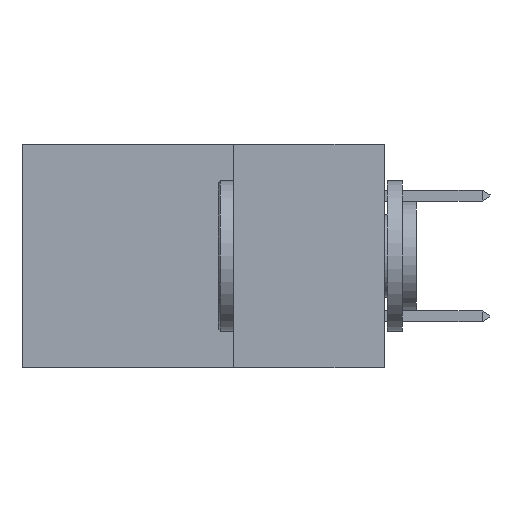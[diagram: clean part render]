
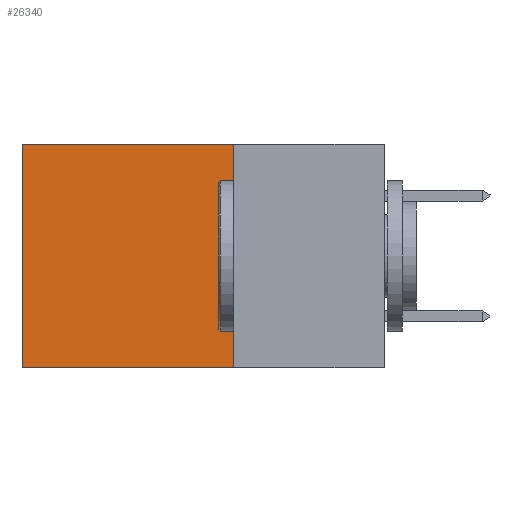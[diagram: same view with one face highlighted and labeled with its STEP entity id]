
A CAD part, left-side view. The second image highlights one B-rep face of the part: STEP entity #26340.
In plain terms, the highlighted planar face has unit normal (-1, 0, 0).
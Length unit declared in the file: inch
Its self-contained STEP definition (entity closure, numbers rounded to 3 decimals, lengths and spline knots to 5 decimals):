
#1391 = ORIENTED_EDGE ( 'NONE', *, *, #42242, .T. ) ;
#2242 = EDGE_CURVE ( 'NONE', #25722, #9152, #29627, .T. ) ;
#4701 = VERTEX_POINT ( 'NONE', #9840 ) ;
#5343 = LINE ( 'NONE', #41043, #11715 ) ;
#8601 = CARTESIAN_POINT ( 'NONE',  ( 0.2875, 0.25, 0. ) ) ;
#9152 = VERTEX_POINT ( 'NONE', #22687 ) ;
#9709 = ORIENTED_EDGE ( 'NONE', *, *, #24052, .T. ) ;
#9840 = CARTESIAN_POINT ( 'NONE',  ( 0.2875, 0.6, 0. ) ) ;
#11491 = LINE ( 'NONE', #37226, #20001 ) ;
#11715 = VECTOR ( 'NONE', #41492, 39.37008 ) ;
#12660 = PLANE ( 'NONE',  #43777 ) ;
#14499 = DIRECTION ( 'NONE',  ( 0., 0., -1. ) ) ;
#16804 = DIRECTION ( 'NONE',  ( 0., 1., 0. ) ) ;
#17143 = CARTESIAN_POINT ( 'NONE',  ( 0.2875, 0.6, -0.37 ) ) ;
#17371 = VECTOR ( 'NONE', #18673, 39.37008 ) ;
#18673 = DIRECTION ( 'NONE',  ( 0., 0., -1. ) ) ;
#20001 = VECTOR ( 'NONE', #16804, 39.37008 ) ;
#20352 = VECTOR ( 'NONE', #14499, 39.37008 ) ;
#20816 = ORIENTED_EDGE ( 'NONE', *, *, #29708, .F. ) ;
#22687 = CARTESIAN_POINT ( 'NONE',  ( 0.2875, 0.25, -0.37 ) ) ;
#24012 = FACE_OUTER_BOUND ( 'NONE', #32135, .T. ) ;
#24052 = EDGE_CURVE ( 'NONE', #25722, #4701, #11491, .T. ) ;
#24263 = CARTESIAN_POINT ( 'NONE',  ( 0.2875, 0.25, 0. ) ) ;
#25722 = VERTEX_POINT ( 'NONE', #24263 ) ;
#26179 = DIRECTION ( 'NONE',  ( 0., 0., -1. ) ) ;
#26340 = ADVANCED_FACE ( 'NONE', ( #24012 ), #12660, .F. ) ;
#29627 = LINE ( 'NONE', #8601, #17371 ) ;
#29708 = EDGE_CURVE ( 'NONE', #9152, #36677, #5343, .T. ) ;
#32135 = EDGE_LOOP ( 'NONE', ( #1391, #20816, #39590, #9709 ) ) ;
#32897 = CARTESIAN_POINT ( 'NONE',  ( 0.2875, 0.25, 0. ) ) ;
#35070 = CARTESIAN_POINT ( 'NONE',  ( 0.2875, 0.6, 0. ) ) ;
#36677 = VERTEX_POINT ( 'NONE', #17143 ) ;
#37226 = CARTESIAN_POINT ( 'NONE',  ( 0.2875, 0.25, 0. ) ) ;
#39590 = ORIENTED_EDGE ( 'NONE', *, *, #2242, .F. ) ;
#41043 = CARTESIAN_POINT ( 'NONE',  ( 0.2875, 0.25, -0.37 ) ) ;
#41492 = DIRECTION ( 'NONE',  ( 0., 1., 0. ) ) ;
#42242 = EDGE_CURVE ( 'NONE', #4701, #36677, #43850, .T. ) ;
#43659 = DIRECTION ( 'NONE',  ( 1., 0., 0. ) ) ;
#43777 = AXIS2_PLACEMENT_3D ( 'NONE', #32897, #43659, #26179 ) ;
#43850 = LINE ( 'NONE', #35070, #20352 ) ;
